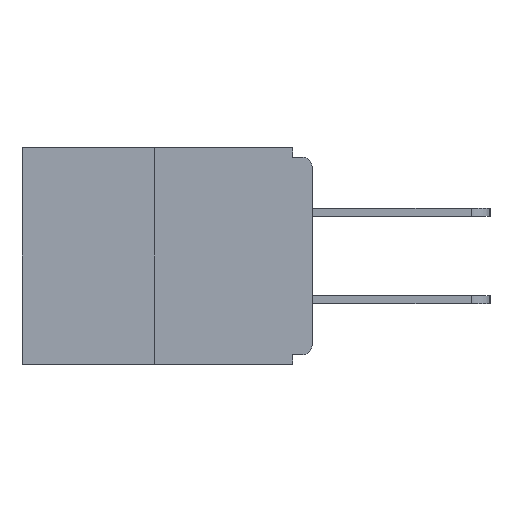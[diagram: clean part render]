
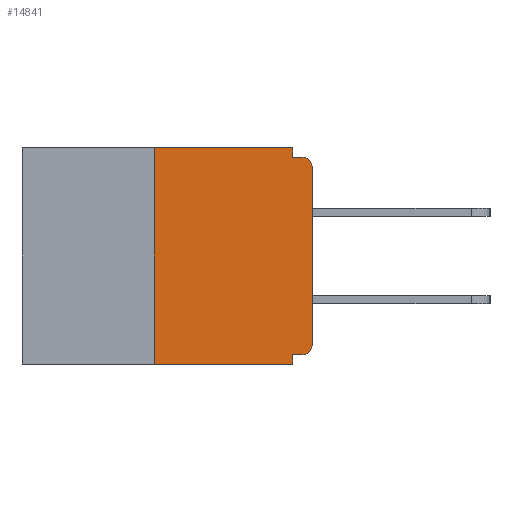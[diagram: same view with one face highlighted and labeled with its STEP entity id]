
A CAD part, left-side view. The second image highlights one B-rep face of the part: STEP entity #14841.
In plain terms, the highlighted planar face has unit normal (-1, 0, 0).
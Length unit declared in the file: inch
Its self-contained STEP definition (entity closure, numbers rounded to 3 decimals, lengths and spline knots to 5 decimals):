
#385 = EDGE_CURVE ( 'NONE', #18530, #6707, #7727, .T. ) ;
#489 = VECTOR ( 'NONE', #10153, 39.37008 ) ;
#754 = CARTESIAN_POINT ( 'NONE',  ( 0., 0.015, -0.03 ) ) ;
#883 = DIRECTION ( 'NONE',  ( -1., 0., 0. ) ) ;
#898 = VECTOR ( 'NONE', #8528, 39.37008 ) ;
#1399 = CARTESIAN_POINT ( 'NONE',  ( 0., 0., -0.328 ) ) ;
#1575 = ORIENTED_EDGE ( 'NONE', *, *, #2476, .T. ) ;
#1605 = ORIENTED_EDGE ( 'NONE', *, *, #8596, .F. ) ;
#1733 = CARTESIAN_POINT ( 'NONE',  ( 0., 0.031, -0.015 ) ) ;
#2283 = VERTEX_POINT ( 'NONE', #14183 ) ;
#2476 = EDGE_CURVE ( 'NONE', #6551, #2283, #2914, .T. ) ;
#2805 = VERTEX_POINT ( 'NONE', #1733 ) ;
#2914 = LINE ( 'NONE', #12629, #13985 ) ;
#3070 = VECTOR ( 'NONE', #3986, 39.37008 ) ;
#3084 = VERTEX_POINT ( 'NONE', #3862 ) ;
#3862 = CARTESIAN_POINT ( 'NONE',  ( 0., 0.015, -0.015 ) ) ;
#3949 = CARTESIAN_POINT ( 'NONE',  ( 0., 0.031, 0. ) ) ;
#3986 = DIRECTION ( 'NONE',  ( 0., 0., -1. ) ) ;
#4185 = CIRCLE ( 'NONE', #13364, 0.015 ) ;
#4738 = EDGE_CURVE ( 'NONE', #8308, #6551, #4185, .T. ) ;
#4859 = DIRECTION ( 'NONE',  ( 0., -1., 0. ) ) ;
#5189 = EDGE_CURVE ( 'NONE', #2805, #3084, #14350, .T. ) ;
#5488 = VECTOR ( 'NONE', #4859, 39.37008 ) ;
#5952 = ORIENTED_EDGE ( 'NONE', *, *, #9697, .T. ) ;
#5967 = VERTEX_POINT ( 'NONE', #3949 ) ;
#6348 = CARTESIAN_POINT ( 'NONE',  ( 0., 0.015, -0.313 ) ) ;
#6400 = DIRECTION ( 'NONE',  ( 0., -1., 0. ) ) ;
#6551 = VERTEX_POINT ( 'NONE', #10096 ) ;
#6553 = FACE_OUTER_BOUND ( 'NONE', #7014, .T. ) ;
#6707 = VERTEX_POINT ( 'NONE', #17476 ) ;
#6915 = AXIS2_PLACEMENT_3D ( 'NONE', #754, #883, #12540 ) ;
#6946 = LINE ( 'NONE', #15600, #3070 ) ;
#7014 = EDGE_LOOP ( 'NONE', ( #18076, #1605, #14767, #10705, #11520, #10790, #1575, #5952, #13990, #15674 ) ) ;
#7616 = DIRECTION ( 'NONE',  ( -1., 0., 0. ) ) ;
#7727 = LINE ( 'NONE', #15692, #898 ) ;
#7957 = VERTEX_POINT ( 'NONE', #16554 ) ;
#8308 = VERTEX_POINT ( 'NONE', #17122 ) ;
#8511 = LINE ( 'NONE', #10911, #12752 ) ;
#8528 = DIRECTION ( 'NONE',  ( 0., -1., 0. ) ) ;
#8550 = CARTESIAN_POINT ( 'NONE',  ( 0., 0.46, 0. ) ) ;
#8596 = EDGE_CURVE ( 'NONE', #18530, #7957, #14466, .T. ) ;
#8782 = DIRECTION ( 'NONE',  ( 0., 0., -1. ) ) ;
#8923 = AXIS2_PLACEMENT_3D ( 'NONE', #8550, #16906, #8782 ) ;
#9697 = EDGE_CURVE ( 'NONE', #2283, #3084, #15537, .T. ) ;
#10096 = CARTESIAN_POINT ( 'NONE',  ( 0., 0., -0.313 ) ) ;
#10153 = DIRECTION ( 'NONE',  ( 0., 1., 0. ) ) ;
#10469 = LINE ( 'NONE', #13444, #5488 ) ;
#10616 = VECTOR ( 'NONE', #16141, 39.37008 ) ;
#10705 = ORIENTED_EDGE ( 'NONE', *, *, #16408, .F. ) ;
#10747 = CARTESIAN_POINT ( 'NONE',  ( 0., 0., -0.015 ) ) ;
#10790 = ORIENTED_EDGE ( 'NONE', *, *, #4738, .T. ) ;
#10842 = EDGE_CURVE ( 'NONE', #5967, #2805, #8511, .T. ) ;
#10911 = CARTESIAN_POINT ( 'NONE',  ( 0., 0.031, 0. ) ) ;
#11520 = ORIENTED_EDGE ( 'NONE', *, *, #17368, .F. ) ;
#11779 = CARTESIAN_POINT ( 'NONE',  ( 0., 0.25, 0. ) ) ;
#11792 = CARTESIAN_POINT ( 'NONE',  ( 0., 0.25, -0.343 ) ) ;
#12228 = DIRECTION ( 'NONE',  ( 0., 0., -1. ) ) ;
#12537 = CARTESIAN_POINT ( 'NONE',  ( 0., 0.031, -0.328 ) ) ;
#12540 = DIRECTION ( 'NONE',  ( 0., 0., -1. ) ) ;
#12629 = CARTESIAN_POINT ( 'NONE',  ( 0., 0., 0. ) ) ;
#12752 = VECTOR ( 'NONE', #12228, 39.37008 ) ;
#13116 = VERTEX_POINT ( 'NONE', #12537 ) ;
#13195 = EDGE_CURVE ( 'NONE', #7957, #5967, #10469, .T. ) ;
#13364 = AXIS2_PLACEMENT_3D ( 'NONE', #6348, #7616, #16251 ) ;
#13444 = CARTESIAN_POINT ( 'NONE',  ( 0., 0.46, 0. ) ) ;
#13985 = VECTOR ( 'NONE', #18490, 39.37008 ) ;
#13990 = ORIENTED_EDGE ( 'NONE', *, *, #5189, .F. ) ;
#14183 = CARTESIAN_POINT ( 'NONE',  ( 0., 0., -0.03 ) ) ;
#14350 = LINE ( 'NONE', #10747, #15924 ) ;
#14466 = LINE ( 'NONE', #11779, #10616 ) ;
#14767 = ORIENTED_EDGE ( 'NONE', *, *, #385, .T. ) ;
#14841 = ADVANCED_FACE ( 'NONE', ( #6553 ), #15715, .F. ) ;
#15537 = CIRCLE ( 'NONE', #6915, 0.015 ) ;
#15600 = CARTESIAN_POINT ( 'NONE',  ( 0., 0.031, -0.343 ) ) ;
#15674 = ORIENTED_EDGE ( 'NONE', *, *, #10842, .F. ) ;
#15692 = CARTESIAN_POINT ( 'NONE',  ( 0., 0.46, -0.343 ) ) ;
#15715 = PLANE ( 'NONE',  #8923 ) ;
#15924 = VECTOR ( 'NONE', #6400, 39.37008 ) ;
#16141 = DIRECTION ( 'NONE',  ( 0., 0., 1. ) ) ;
#16251 = DIRECTION ( 'NONE',  ( 0., 0., -1. ) ) ;
#16408 = EDGE_CURVE ( 'NONE', #13116, #6707, #6946, .T. ) ;
#16554 = CARTESIAN_POINT ( 'NONE',  ( 0., 0.25, 0. ) ) ;
#16870 = LINE ( 'NONE', #1399, #489 ) ;
#16906 = DIRECTION ( 'NONE',  ( 1., 0., 0. ) ) ;
#17122 = CARTESIAN_POINT ( 'NONE',  ( 0., 0.015, -0.328 ) ) ;
#17368 = EDGE_CURVE ( 'NONE', #8308, #13116, #16870, .T. ) ;
#17476 = CARTESIAN_POINT ( 'NONE',  ( 0., 0.031, -0.343 ) ) ;
#18076 = ORIENTED_EDGE ( 'NONE', *, *, #13195, .F. ) ;
#18490 = DIRECTION ( 'NONE',  ( 0., 0., 1. ) ) ;
#18530 = VERTEX_POINT ( 'NONE', #11792 ) ;
